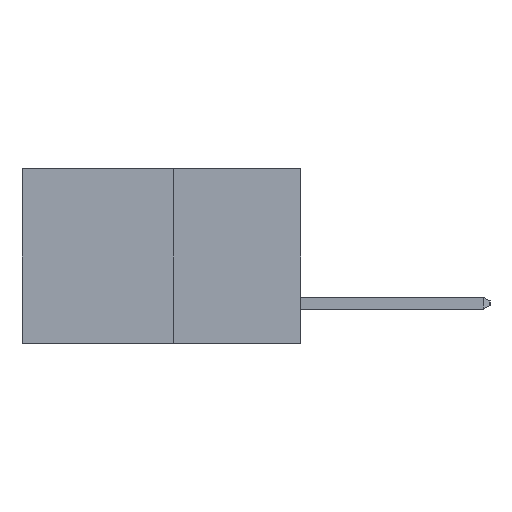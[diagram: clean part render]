
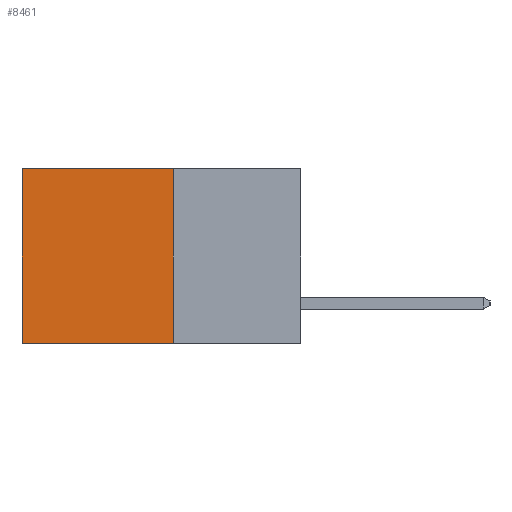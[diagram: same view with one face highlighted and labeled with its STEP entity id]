
A CAD part, left-side view. The second image highlights one B-rep face of the part: STEP entity #8461.
In plain terms, the highlighted planar face has unit normal (-1, 0, 0).
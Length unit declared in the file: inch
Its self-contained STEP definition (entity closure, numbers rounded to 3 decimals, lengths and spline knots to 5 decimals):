
#69 = VECTOR ( 'NONE', #11715, 39.37008 ) ;
#224 = ORIENTED_EDGE ( 'NONE', *, *, #6429, .F. ) ;
#315 = FACE_OUTER_BOUND ( 'NONE', #1004, .T. ) ;
#1004 = EDGE_LOOP ( 'NONE', ( #5180, #2994, #224, #8363 ) ) ;
#1522 = CARTESIAN_POINT ( 'NONE',  ( 0.277, 0.59, -0.37 ) ) ;
#2149 = EDGE_CURVE ( 'NONE', #14760, #6387, #14478, .T. ) ;
#2532 = CARTESIAN_POINT ( 'NONE',  ( 0.277, 0.27, 0. ) ) ;
#2634 = LINE ( 'NONE', #1522, #9610 ) ;
#2675 = AXIS2_PLACEMENT_3D ( 'NONE', #13335, #14636, #6806 ) ;
#2994 = ORIENTED_EDGE ( 'NONE', *, *, #2149, .F. ) ;
#3620 = VERTEX_POINT ( 'NONE', #14022 ) ;
#5180 = ORIENTED_EDGE ( 'NONE', *, *, #15383, .T. ) ;
#6387 = VERTEX_POINT ( 'NONE', #10729 ) ;
#6429 = EDGE_CURVE ( 'NONE', #3620, #14760, #15141, .T. ) ;
#6806 = DIRECTION ( 'NONE',  ( 0., 0., -1. ) ) ;
#7015 = VERTEX_POINT ( 'NONE', #15821 ) ;
#7062 = LINE ( 'NONE', #2532, #69 ) ;
#7464 = DIRECTION ( 'NONE',  ( 0., 1., 0. ) ) ;
#8168 = VECTOR ( 'NONE', #9774, 39.37008 ) ;
#8363 = ORIENTED_EDGE ( 'NONE', *, *, #11714, .T. ) ;
#8461 = ADVANCED_FACE ( 'NONE', ( #315 ), #12032, .F. ) ;
#9610 = VECTOR ( 'NONE', #13345, 39.37008 ) ;
#9774 = DIRECTION ( 'NONE',  ( 0., 0., -1. ) ) ;
#10116 = CARTESIAN_POINT ( 'NONE',  ( 0.277, 0.27, -0.37 ) ) ;
#10609 = VECTOR ( 'NONE', #7464, 39.37008 ) ;
#10729 = CARTESIAN_POINT ( 'NONE',  ( 0.277, 0.59, -0.37 ) ) ;
#10749 = CARTESIAN_POINT ( 'NONE',  ( 0.277, 0.27, -0.37 ) ) ;
#10929 = CARTESIAN_POINT ( 'NONE',  ( 0.277, 0.27, -0.37 ) ) ;
#11714 = EDGE_CURVE ( 'NONE', #3620, #7015, #7062, .T. ) ;
#11715 = DIRECTION ( 'NONE',  ( 0., 1., 0. ) ) ;
#12032 = PLANE ( 'NONE',  #2675 ) ;
#13335 = CARTESIAN_POINT ( 'NONE',  ( 0.277, 0.27, -0.37 ) ) ;
#13345 = DIRECTION ( 'NONE',  ( 0., 0., -1. ) ) ;
#14022 = CARTESIAN_POINT ( 'NONE',  ( 0.277, 0.27, 0. ) ) ;
#14478 = LINE ( 'NONE', #10929, #10609 ) ;
#14636 = DIRECTION ( 'NONE',  ( 1., 0., 0. ) ) ;
#14760 = VERTEX_POINT ( 'NONE', #10749 ) ;
#15141 = LINE ( 'NONE', #10116, #8168 ) ;
#15383 = EDGE_CURVE ( 'NONE', #7015, #6387, #2634, .T. ) ;
#15821 = CARTESIAN_POINT ( 'NONE',  ( 0.277, 0.59, 0. ) ) ;
